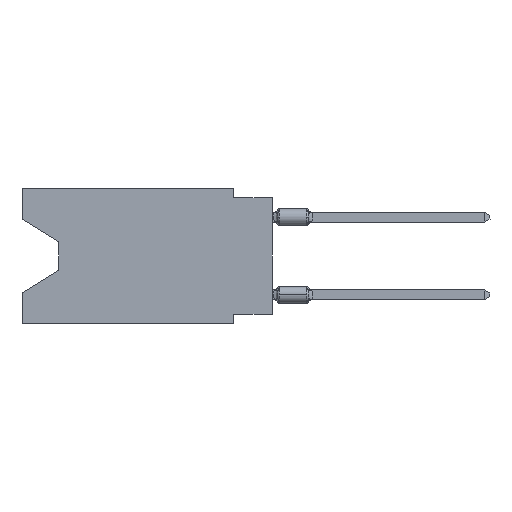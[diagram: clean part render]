
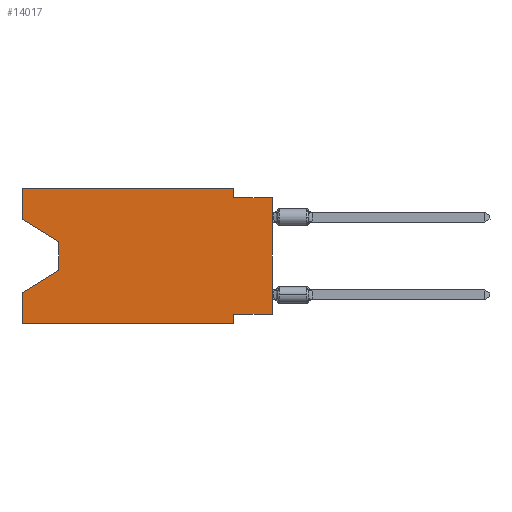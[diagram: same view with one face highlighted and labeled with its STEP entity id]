
A CAD part, left-side view. The second image highlights one B-rep face of the part: STEP entity #14017.
In plain terms, the highlighted planar face has unit normal (-1, 0, 0).
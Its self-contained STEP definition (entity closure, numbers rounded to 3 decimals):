
#325 = PLANE ( 'NONE',  #4048 ) ;
#396 = VECTOR ( 'NONE', #13025, 1000. ) ;
#401 = LINE ( 'NONE', #13073, #2742 ) ;
#699 = ORIENTED_EDGE ( 'NONE', *, *, #2237, .T. ) ;
#726 = VERTEX_POINT ( 'NONE', #14129 ) ;
#868 = ORIENTED_EDGE ( 'NONE', *, *, #4415, .T. ) ;
#967 = VECTOR ( 'NONE', #8480, 1000. ) ;
#977 = CARTESIAN_POINT ( 'NONE',  ( 0., 0., 0. ) ) ;
#1117 = DIRECTION ( 'NONE',  ( 0., -1., 0. ) ) ;
#1126 = VECTOR ( 'NONE', #4429, 1000. ) ;
#1364 = CARTESIAN_POINT ( 'NONE',  ( 0., 16.383, 0. ) ) ;
#1425 = EDGE_CURVE ( 'NONE', #9334, #1688, #3522, .T. ) ;
#1688 = VERTEX_POINT ( 'NONE', #14410 ) ;
#2081 = ORIENTED_EDGE ( 'NONE', *, *, #9854, .F. ) ;
#2098 = DIRECTION ( 'NONE',  ( 0., -0.855, -0.519 ) ) ;
#2237 = EDGE_CURVE ( 'NONE', #13764, #15576, #5908, .T. ) ;
#2290 = LINE ( 'NONE', #1364, #6821 ) ;
#2327 = EDGE_CURVE ( 'NONE', #11284, #8626, #2290, .T. ) ;
#2624 = VECTOR ( 'NONE', #2098, 1000. ) ;
#2742 = VECTOR ( 'NONE', #15779, 1000. ) ;
#3131 = VECTOR ( 'NONE', #14356, 1000. ) ;
#3378 = LINE ( 'NONE', #10908, #8476 ) ;
#3522 = LINE ( 'NONE', #8633, #2624 ) ;
#3592 = ORIENTED_EDGE ( 'NONE', *, *, #11466, .F. ) ;
#3819 = CARTESIAN_POINT ( 'NONE',  ( 0., 16.383, -2.038 ) ) ;
#4023 = EDGE_CURVE ( 'NONE', #726, #15576, #3378, .T. ) ;
#4048 = AXIS2_PLACEMENT_3D ( 'NONE', #7817, #7981, #14429 ) ;
#4079 = VECTOR ( 'NONE', #12733, 1000. ) ;
#4143 = ORIENTED_EDGE ( 'NONE', *, *, #8212, .F. ) ;
#4311 = LINE ( 'NONE', #15572, #396 ) ;
#4415 = EDGE_CURVE ( 'NONE', #1688, #13764, #14937, .T. ) ;
#4429 = DIRECTION ( 'NONE',  ( 0., -1., 0. ) ) ;
#4539 = CARTESIAN_POINT ( 'NONE',  ( 0., 2.54, -8.255 ) ) ;
#4545 = CARTESIAN_POINT ( 'NONE',  ( 0., 0., -8.255 ) ) ;
#5576 = VERTEX_POINT ( 'NONE', #4539 ) ;
#5634 = CARTESIAN_POINT ( 'NONE',  ( 0., 13.97, -3.505 ) ) ;
#5715 = LINE ( 'NONE', #14864, #12875 ) ;
#5834 = VECTOR ( 'NONE', #12555, 1000. ) ;
#5894 = DIRECTION ( 'NONE',  ( 0., 0., 1. ) ) ;
#5908 = LINE ( 'NONE', #12102, #15377 ) ;
#6821 = VECTOR ( 'NONE', #1117, 1000. ) ;
#7198 = CARTESIAN_POINT ( 'NONE',  ( 0., 2.54, -0.635 ) ) ;
#7368 = LINE ( 'NONE', #977, #5834 ) ;
#7408 = ORIENTED_EDGE ( 'NONE', *, *, #4023, .F. ) ;
#7817 = CARTESIAN_POINT ( 'NONE',  ( 0., 16.383, 0. ) ) ;
#7863 = ORIENTED_EDGE ( 'NONE', *, *, #11520, .F. ) ;
#7981 = DIRECTION ( 'NONE',  ( 1., 0., 0. ) ) ;
#8026 = ORIENTED_EDGE ( 'NONE', *, *, #2327, .F. ) ;
#8209 = CARTESIAN_POINT ( 'NONE',  ( 0., 0., -0.635 ) ) ;
#8212 = EDGE_CURVE ( 'NONE', #10070, #5576, #4311, .T. ) ;
#8310 = CARTESIAN_POINT ( 'NONE',  ( 0., 2.54, -8.89 ) ) ;
#8476 = VECTOR ( 'NONE', #5894, 1000. ) ;
#8480 = DIRECTION ( 'NONE',  ( 0., 0., -1. ) ) ;
#8491 = DIRECTION ( 'NONE',  ( 0., 0., -1. ) ) ;
#8595 = ORIENTED_EDGE ( 'NONE', *, *, #1425, .T. ) ;
#8626 = VERTEX_POINT ( 'NONE', #14505 ) ;
#8628 = VERTEX_POINT ( 'NONE', #8310 ) ;
#8633 = CARTESIAN_POINT ( 'NONE',  ( 0., 16.383, -2.038 ) ) ;
#9239 = CARTESIAN_POINT ( 'NONE',  ( 0., 2.54, -8.89 ) ) ;
#9255 = VERTEX_POINT ( 'NONE', #7198 ) ;
#9334 = VERTEX_POINT ( 'NONE', #3819 ) ;
#9854 = EDGE_CURVE ( 'NONE', #5576, #8628, #11829, .T. ) ;
#10070 = VERTEX_POINT ( 'NONE', #4545 ) ;
#10393 = VERTEX_POINT ( 'NONE', #8209 ) ;
#10786 = EDGE_LOOP ( 'NONE', ( #8595, #868, #699, #7408, #10836, #2081, #4143, #12916, #3592, #16161, #8026, #7863 ) ) ;
#10797 = CARTESIAN_POINT ( 'NONE',  ( 0., 0., -0.635 ) ) ;
#10836 = ORIENTED_EDGE ( 'NONE', *, *, #11241, .T. ) ;
#10908 = CARTESIAN_POINT ( 'NONE',  ( 0., 16.383, 0. ) ) ;
#11008 = DIRECTION ( 'NONE',  ( 0., 0.855, -0.519 ) ) ;
#11241 = EDGE_CURVE ( 'NONE', #726, #8628, #15883, .T. ) ;
#11284 = VERTEX_POINT ( 'NONE', #12821 ) ;
#11466 = EDGE_CURVE ( 'NONE', #9255, #10393, #15862, .T. ) ;
#11520 = EDGE_CURVE ( 'NONE', #9334, #11284, #401, .T. ) ;
#11829 = LINE ( 'NONE', #9239, #3131 ) ;
#11898 = FACE_OUTER_BOUND ( 'NONE', #10786, .T. ) ;
#12102 = CARTESIAN_POINT ( 'NONE',  ( 0., 13.97, -5.385 ) ) ;
#12131 = CARTESIAN_POINT ( 'NONE',  ( 0., 16.383, -6.852 ) ) ;
#12555 = DIRECTION ( 'NONE',  ( 0., 0., 1. ) ) ;
#12733 = DIRECTION ( 'NONE',  ( 0., -1., 0. ) ) ;
#12821 = CARTESIAN_POINT ( 'NONE',  ( 0., 16.383, 0. ) ) ;
#12875 = VECTOR ( 'NONE', #8491, 1000. ) ;
#12916 = ORIENTED_EDGE ( 'NONE', *, *, #15787, .T. ) ;
#13025 = DIRECTION ( 'NONE',  ( 0., 1., 0. ) ) ;
#13073 = CARTESIAN_POINT ( 'NONE',  ( 0., 16.383, 0. ) ) ;
#13516 = CARTESIAN_POINT ( 'NONE',  ( 0., 13.97, -5.385 ) ) ;
#13764 = VERTEX_POINT ( 'NONE', #13516 ) ;
#13802 = EDGE_CURVE ( 'NONE', #8626, #9255, #5715, .T. ) ;
#14017 = ADVANCED_FACE ( 'NONE', ( #11898 ), #325, .F. ) ;
#14129 = CARTESIAN_POINT ( 'NONE',  ( 0., 16.383, -8.89 ) ) ;
#14356 = DIRECTION ( 'NONE',  ( 0., 0., -1. ) ) ;
#14410 = CARTESIAN_POINT ( 'NONE',  ( 0., 13.97, -3.505 ) ) ;
#14429 = DIRECTION ( 'NONE',  ( 0., 0., -1. ) ) ;
#14505 = CARTESIAN_POINT ( 'NONE',  ( 0., 2.54, 0. ) ) ;
#14864 = CARTESIAN_POINT ( 'NONE',  ( 0., 2.54, 0. ) ) ;
#14937 = LINE ( 'NONE', #5634, #967 ) ;
#15274 = CARTESIAN_POINT ( 'NONE',  ( 0., 16.383, -8.89 ) ) ;
#15377 = VECTOR ( 'NONE', #11008, 1000. ) ;
#15572 = CARTESIAN_POINT ( 'NONE',  ( 0., 0., -8.255 ) ) ;
#15576 = VERTEX_POINT ( 'NONE', #12131 ) ;
#15779 = DIRECTION ( 'NONE',  ( 0., 0., 1. ) ) ;
#15787 = EDGE_CURVE ( 'NONE', #10070, #10393, #7368, .T. ) ;
#15862 = LINE ( 'NONE', #10797, #1126 ) ;
#15883 = LINE ( 'NONE', #15274, #4079 ) ;
#16161 = ORIENTED_EDGE ( 'NONE', *, *, #13802, .F. ) ;
